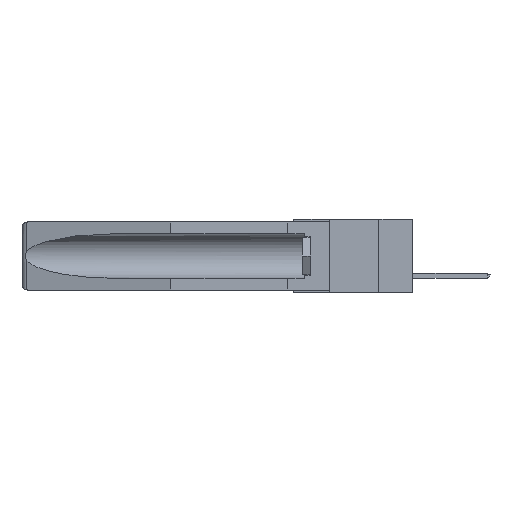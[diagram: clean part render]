
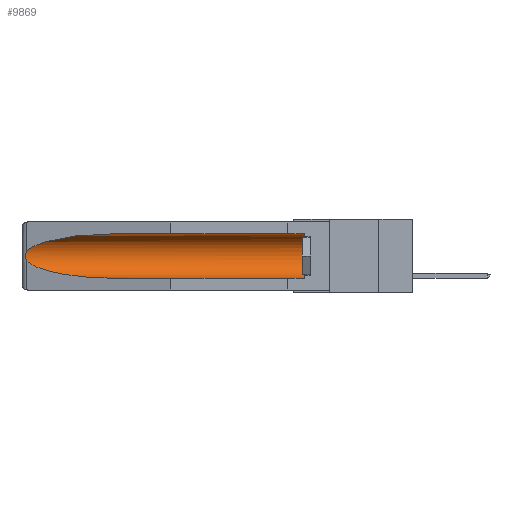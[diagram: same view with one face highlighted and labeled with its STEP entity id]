
A CAD part, left-side view. The second image highlights one B-rep face of the part: STEP entity #9869.
In plain terms, the highlighted cylindrical face has radius 2.857 mm (diameter 5.715 mm), a partial arc.
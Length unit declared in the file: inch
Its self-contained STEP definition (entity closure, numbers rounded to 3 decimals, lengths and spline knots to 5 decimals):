
#109 = CIRCLE ( 'NONE', #24206, 0.1125 ) ;
#1530 = CARTESIAN_POINT ( 'NONE',  ( 0.26537, 1.52718, -0.14972 ) ) ;
#1578 = VECTOR ( 'NONE', #1739, 39.37008 ) ;
#1739 = DIRECTION ( 'NONE',  ( 0., 1., 0. ) ) ;
#2340 = EDGE_CURVE ( 'NONE', #23986, #22797, #109, .T. ) ;
#2680 = DIRECTION ( 'NONE',  ( 0., 0., 1. ) ) ;
#2870 =( BOUNDED_CURVE ( )  B_SPLINE_CURVE ( 3, ( #16013, #17947, #10230, #16351 ),
 .UNSPECIFIED., .F., .F. ) 
 B_SPLINE_CURVE_WITH_KNOTS ( ( 4, 4 ),
 ( 4.71239, 6.08839 ),
 .UNSPECIFIED. ) 
 CURVE ( )  GEOMETRIC_REPRESENTATION_ITEM ( )  RATIONAL_B_SPLINE_CURVE ( ( 1., 0.848, 0.848, 1. ) ) 
 REPRESENTATION_ITEM ( '' )  );
#3145 = CARTESIAN_POINT ( 'NONE',  ( 0.26597, 1.52961, -0.15275 ) ) ;
#3227 = ORIENTED_EDGE ( 'NONE', *, *, #2340, .T. ) ;
#3477 = CARTESIAN_POINT ( 'NONE',  ( 0.2673, 1.53269, -0.17917 ) ) ;
#4765 = ORIENTED_EDGE ( 'NONE', *, *, #14938, .T. ) ;
#5367 = CARTESIAN_POINT ( 'NONE',  ( 0.2675, 1.53308, -0.17534 ) ) ;
#5867 = LINE ( 'NONE', #15080, #1578 ) ;
#5944 = CARTESIAN_POINT ( 'NONE',  ( 0.155, 0.126, -0.284 ) ) ;
#6301 = B_SPLINE_CURVE_WITH_KNOTS ( 'NONE', 3,
 ( #1530, #3145, #7240, #18710, #24513, #5367, #3477, #24859, #11171, #9200 ),
 .UNSPECIFIED., .F., .F.,
 ( 4, 2, 2, 2, 4 ),
 ( 0., 0.00029, 0.00058, 0.00087, 0.00117 ),
 .UNSPECIFIED. ) ;
#6318 = EDGE_CURVE ( 'NONE', #21343, #17902, #12272, .T. ) ;
#7240 = CARTESIAN_POINT ( 'NONE',  ( 0.26654, 1.53092, -0.15636 ) ) ;
#8204 = ORIENTED_EDGE ( 'NONE', *, *, #6318, .T. ) ;
#8950 = CARTESIAN_POINT ( 'NONE',  ( 0.155, 1.07973, -0.284 ) ) ;
#9200 = CARTESIAN_POINT ( 'NONE',  ( 0.26537, 1.52718, -0.19328 ) ) ;
#9869 = ADVANCED_FACE ( 'NONE', ( #24098 ), #24714, .F. ) ;
#10230 = CARTESIAN_POINT ( 'NONE',  ( 0.25451, 1.48313, -0.09465 ) ) ;
#10643 = DIRECTION ( 'NONE',  ( 0., 1., 0. ) ) ;
#11171 = CARTESIAN_POINT ( 'NONE',  ( 0.26597, 1.5296, -0.19026 ) ) ;
#11995 = CARTESIAN_POINT ( 'NONE',  ( 0.26537, 1.52718, -0.14972 ) ) ;
#12272 =( BOUNDED_CURVE ( )  B_SPLINE_CURVE ( 3, ( #24051, #12412, #20339, #16487 ),
 .UNSPECIFIED., .F., .F. ) 
 B_SPLINE_CURVE_WITH_KNOTS ( ( 4, 4 ),
 ( 0.1948, 1.5708 ),
 .UNSPECIFIED. ) 
 CURVE ( )  GEOMETRIC_REPRESENTATION_ITEM ( )  RATIONAL_B_SPLINE_CURVE ( ( 1., 0.848, 0.848, 1. ) ) 
 REPRESENTATION_ITEM ( '' )  );
#12336 = CARTESIAN_POINT ( 'NONE',  ( 0.155, -0.30754, -0.1715 ) ) ;
#12337 = CARTESIAN_POINT ( 'NONE',  ( 0.155, 1.07973, -0.059 ) ) ;
#12412 = CARTESIAN_POINT ( 'NONE',  ( 0.25451, 1.48313, -0.24835 ) ) ;
#13130 = EDGE_LOOP ( 'NONE', ( #20361, #24322, #8204, #15455, #3227, #4765 ) ) ;
#13269 = EDGE_CURVE ( 'NONE', #24248, #22719, #2870, .T. ) ;
#14472 = DIRECTION ( 'NONE',  ( 0., -1., 0. ) ) ;
#14938 = EDGE_CURVE ( 'NONE', #22797, #24248, #5867, .T. ) ;
#15080 = CARTESIAN_POINT ( 'NONE',  ( 0.155, -0.30754, -0.059 ) ) ;
#15455 = ORIENTED_EDGE ( 'NONE', *, *, #23771, .F. ) ;
#16013 = CARTESIAN_POINT ( 'NONE',  ( 0.155, 1.07973, -0.059 ) ) ;
#16240 = DIRECTION ( 'NONE',  ( 0., 1., 0. ) ) ;
#16351 = CARTESIAN_POINT ( 'NONE',  ( 0.26537, 1.52718, -0.14972 ) ) ;
#16487 = CARTESIAN_POINT ( 'NONE',  ( 0.155, 1.07973, -0.284 ) ) ;
#17510 = CARTESIAN_POINT ( 'NONE',  ( 0.26537, 1.52718, -0.19328 ) ) ;
#17902 = VERTEX_POINT ( 'NONE', #8950 ) ;
#17947 = CARTESIAN_POINT ( 'NONE',  ( 0.21114, 1.30732, -0.059 ) ) ;
#17995 = DIRECTION ( 'NONE',  ( 0., 0., 1. ) ) ;
#18710 = CARTESIAN_POINT ( 'NONE',  ( 0.2673, 1.5327, -0.16383 ) ) ;
#19264 = VECTOR ( 'NONE', #10643, 39.37008 ) ;
#20339 = CARTESIAN_POINT ( 'NONE',  ( 0.21114, 1.30732, -0.284 ) ) ;
#20361 = ORIENTED_EDGE ( 'NONE', *, *, #13269, .T. ) ;
#21024 = CARTESIAN_POINT ( 'NONE',  ( 0.155, 0.126, -0.059 ) ) ;
#21094 = AXIS2_PLACEMENT_3D ( 'NONE', #12336, #16240, #17995 ) ;
#21343 = VERTEX_POINT ( 'NONE', #17510 ) ;
#22165 = CARTESIAN_POINT ( 'NONE',  ( 0.155, 0.126, -0.1715 ) ) ;
#22719 = VERTEX_POINT ( 'NONE', #11995 ) ;
#22797 = VERTEX_POINT ( 'NONE', #21024 ) ;
#23289 = EDGE_CURVE ( 'NONE', #22719, #21343, #6301, .T. ) ;
#23771 = EDGE_CURVE ( 'NONE', #23986, #17902, #24454, .T. ) ;
#23986 = VERTEX_POINT ( 'NONE', #5944 ) ;
#24051 = CARTESIAN_POINT ( 'NONE',  ( 0.26537, 1.52718, -0.19328 ) ) ;
#24098 = FACE_OUTER_BOUND ( 'NONE', #13130, .T. ) ;
#24206 = AXIS2_PLACEMENT_3D ( 'NONE', #22165, #14472, #2680 ) ;
#24248 = VERTEX_POINT ( 'NONE', #12337 ) ;
#24322 = ORIENTED_EDGE ( 'NONE', *, *, #23289, .T. ) ;
#24454 = LINE ( 'NONE', #24921, #19264 ) ;
#24513 = CARTESIAN_POINT ( 'NONE',  ( 0.2675, 1.53308, -0.16763 ) ) ;
#24714 = CYLINDRICAL_SURFACE ( 'NONE', #21094, 0.1125 ) ;
#24859 = CARTESIAN_POINT ( 'NONE',  ( 0.26655, 1.53094, -0.18657 ) ) ;
#24921 = CARTESIAN_POINT ( 'NONE',  ( 0.155, -0.30754, -0.284 ) ) ;
